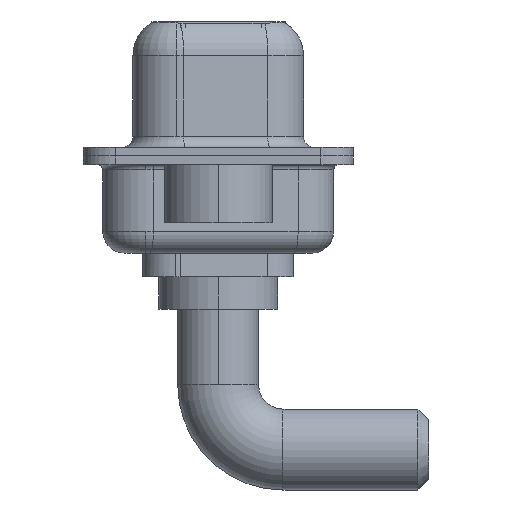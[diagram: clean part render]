
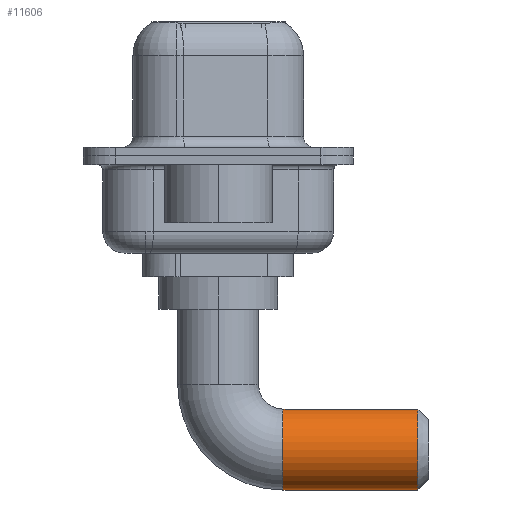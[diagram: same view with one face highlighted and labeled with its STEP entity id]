
A CAD part, left-side view. The second image highlights one B-rep face of the part: STEP entity #11606.
In plain terms, the highlighted cylindrical face has radius 1.875 mm (diameter 3.75 mm), a partial arc.
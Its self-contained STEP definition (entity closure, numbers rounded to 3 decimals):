
#36 = VECTOR ( 'NONE', #8548, 1000. ) ;
#703 = AXIS2_PLACEMENT_3D ( 'NONE', #7952, #3905, #12055 ) ;
#1322 = DIRECTION ( 'NONE',  ( -1., 0., 0. ) ) ;
#1447 = ORIENTED_EDGE ( 'NONE', *, *, #13117, .F. ) ;
#1498 = CARTESIAN_POINT ( 'NONE',  ( 0., -9.25, -4.625 ) ) ;
#1516 = VERTEX_POINT ( 'NONE', #1498 ) ;
#2395 = ORIENTED_EDGE ( 'NONE', *, *, #10237, .T. ) ;
#2819 = CARTESIAN_POINT ( 'NONE',  ( 0., -9.25, -6.5 ) ) ;
#3059 = EDGE_CURVE ( 'NONE', #12635, #1516, #6958, .T. ) ;
#3509 = AXIS2_PLACEMENT_3D ( 'NONE', #2819, #4967, #13188 ) ;
#3599 = VERTEX_POINT ( 'NONE', #8325 ) ;
#3837 = CYLINDRICAL_SURFACE ( 'NONE', #703, 1.875 ) ;
#3905 = DIRECTION ( 'NONE',  ( 0., -1., 0. ) ) ;
#3976 = VECTOR ( 'NONE', #11422, 1000. ) ;
#4834 = CIRCLE ( 'NONE', #10867, 1.875 ) ;
#4967 = DIRECTION ( 'NONE',  ( 0., 1., 0. ) ) ;
#5292 = LINE ( 'NONE', #5541, #3976 ) ;
#5541 = CARTESIAN_POINT ( 'NONE',  ( 0., -3., -4.625 ) ) ;
#5614 = VERTEX_POINT ( 'NONE', #8010 ) ;
#5903 = EDGE_CURVE ( 'NONE', #5614, #3599, #4834, .T. ) ;
#6562 = ORIENTED_EDGE ( 'NONE', *, *, #3059, .T. ) ;
#6958 = CIRCLE ( 'NONE', #3509, 1.875 ) ;
#7952 = CARTESIAN_POINT ( 'NONE',  ( 0., -3., -6.5 ) ) ;
#8010 = CARTESIAN_POINT ( 'NONE',  ( 0., -3., -4.625 ) ) ;
#8325 = CARTESIAN_POINT ( 'NONE',  ( 0., -3., -8.375 ) ) ;
#8348 = LINE ( 'NONE', #9299, #36 ) ;
#8548 = DIRECTION ( 'NONE',  ( 0., -1., 0. ) ) ;
#8673 = DIRECTION ( 'NONE',  ( 0., -1., 0. ) ) ;
#9299 = CARTESIAN_POINT ( 'NONE',  ( 0., -3., -8.375 ) ) ;
#10212 = EDGE_LOOP ( 'NONE', ( #1447, #11163, #2395, #6562 ) ) ;
#10237 = EDGE_CURVE ( 'NONE', #3599, #12635, #8348, .T. ) ;
#10442 = CARTESIAN_POINT ( 'NONE',  ( 0., -3., -6.5 ) ) ;
#10867 = AXIS2_PLACEMENT_3D ( 'NONE', #10442, #8673, #1322 ) ;
#11163 = ORIENTED_EDGE ( 'NONE', *, *, #5903, .T. ) ;
#11422 = DIRECTION ( 'NONE',  ( 0., -1., 0. ) ) ;
#11606 = ADVANCED_FACE ( 'NONE', ( #12130 ), #3837, .T. ) ;
#12055 = DIRECTION ( 'NONE',  ( 0., 0., -1. ) ) ;
#12130 = FACE_OUTER_BOUND ( 'NONE', #10212, .T. ) ;
#12188 = CARTESIAN_POINT ( 'NONE',  ( 0., -9.25, -8.375 ) ) ;
#12635 = VERTEX_POINT ( 'NONE', #12188 ) ;
#13117 = EDGE_CURVE ( 'NONE', #5614, #1516, #5292, .T. ) ;
#13188 = DIRECTION ( 'NONE',  ( 0., 0., -1. ) ) ;
